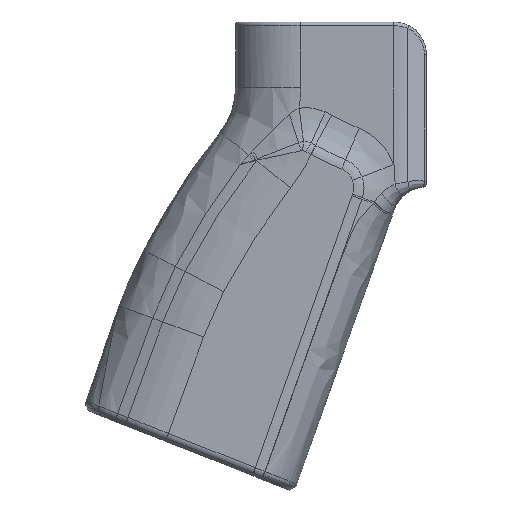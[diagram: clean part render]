
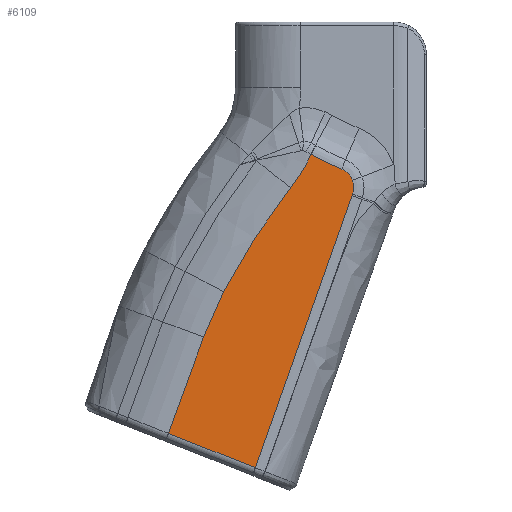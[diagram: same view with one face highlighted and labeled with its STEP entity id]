
A CAD part, left-side view. The second image highlights one B-rep face of the part: STEP entity #6109.
In plain terms, the highlighted planar face has unit normal (-1, 0, 0).
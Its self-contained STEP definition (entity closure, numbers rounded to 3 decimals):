
#480=CIRCLE('',#6562,75.936);
#483=CIRCLE('',#6565,3.889);
#783=FACE_OUTER_BOUND('',#1200,.T.);
#1200=EDGE_LOOP('',(#4482,#4483,#4484,#4485,#4486,#4487,#4488,#4489,#4490,
#4491,#4492,#4493));
#1537=LINE('',#11214,#1730);
#1538=LINE('',#11223,#1731);
#1539=LINE('',#11225,#1732);
#1730=VECTOR('',#7154,10.);
#1731=VECTOR('',#7159,10.);
#1732=VECTOR('',#7160,10.);
#2043=B_SPLINE_CURVE_WITH_KNOTS('',3,(#11066,#11067,#11068,#11069),
 .UNSPECIFIED.,.F.,.F.,(4,4),(-0.965,0.),.UNSPECIFIED.);
#2044=B_SPLINE_CURVE_WITH_KNOTS('',3,(#11088,#11089,#11090,#11091),
 .UNSPECIFIED.,.F.,.F.,(4,4),(-2.413,0.),.UNSPECIFIED.);
#2045=B_SPLINE_CURVE_WITH_KNOTS('',3,(#11109,#11110,#11111,#11112),
 .UNSPECIFIED.,.F.,.F.,(4,4),(-0.596,0.166),
 .UNSPECIFIED.);
#2047=B_SPLINE_CURVE_WITH_KNOTS('',3,(#11156,#11157,#11158,#11159),
 .UNSPECIFIED.,.F.,.F.,(4,4),(0.,0.275),.UNSPECIFIED.);
#2049=B_SPLINE_CURVE_WITH_KNOTS('',3,(#11200,#11201,#11202,#11203),
 .UNSPECIFIED.,.F.,.F.,(4,4),(-0.031,0.),
 .UNSPECIFIED.);
#2052=B_SPLINE_CURVE_WITH_KNOTS('',3,(#11227,#11228,#11229,#11230),
 .UNSPECIFIED.,.F.,.F.,(4,4),(0.,0.002),.UNSPECIFIED.);
#2053=B_SPLINE_CURVE_WITH_KNOTS('',3,(#11231,#11232,#11233,#11234),
 .UNSPECIFIED.,.F.,.F.,(4,4),(0.,0.002),
 .UNSPECIFIED.);
#2586=VERTEX_POINT('',#10744);
#2591=VERTEX_POINT('',#11063);
#2592=VERTEX_POINT('',#11065);
#2593=VERTEX_POINT('',#11087);
#2594=VERTEX_POINT('',#11114);
#2596=VERTEX_POINT('',#11128);
#2599=VERTEX_POINT('',#11150);
#2601=VERTEX_POINT('',#11199);
#2604=VERTEX_POINT('',#11213);
#2606=VERTEX_POINT('',#11222);
#2607=VERTEX_POINT('',#11224);
#2608=VERTEX_POINT('',#11226);
#3273=EDGE_CURVE('',#2591,#2592,#2043,.T.);
#3275=EDGE_CURVE('',#2592,#2593,#2044,.T.);
#3277=EDGE_CURVE('',#2593,#2586,#2045,.T.);
#3278=EDGE_CURVE('',#2586,#2594,#480,.T.);
#3281=EDGE_CURVE('',#2594,#2596,#483,.T.);
#3286=EDGE_CURVE('',#2596,#2599,#2047,.T.);
#3290=EDGE_CURVE('',#2599,#2601,#2049,.T.);
#3294=EDGE_CURVE('',#2601,#2604,#1537,.T.);
#3297=EDGE_CURVE('',#2604,#2606,#1538,.T.);
#3298=EDGE_CURVE('',#2607,#2591,#1539,.T.);
#3299=EDGE_CURVE('',#2608,#2607,#2052,.T.);
#3300=EDGE_CURVE('',#2606,#2608,#2053,.T.);
#4482=ORIENTED_EDGE('',*,*,#3297,.F.);
#4483=ORIENTED_EDGE('',*,*,#3294,.F.);
#4484=ORIENTED_EDGE('',*,*,#3290,.F.);
#4485=ORIENTED_EDGE('',*,*,#3286,.F.);
#4486=ORIENTED_EDGE('',*,*,#3281,.F.);
#4487=ORIENTED_EDGE('',*,*,#3278,.F.);
#4488=ORIENTED_EDGE('',*,*,#3277,.F.);
#4489=ORIENTED_EDGE('',*,*,#3275,.F.);
#4490=ORIENTED_EDGE('',*,*,#3273,.F.);
#4491=ORIENTED_EDGE('',*,*,#3298,.F.);
#4492=ORIENTED_EDGE('',*,*,#3299,.F.);
#4493=ORIENTED_EDGE('',*,*,#3300,.F.);
#5954=PLANE('',#6574);
#6109=ADVANCED_FACE('',(#783),#5954,.T.);
#6562=AXIS2_PLACEMENT_3D('',#11115,#7131,#7132);
#6565=AXIS2_PLACEMENT_3D('',#11129,#7137,#7138);
#6574=AXIS2_PLACEMENT_3D('',#11221,#7157,#7158);
#7131=DIRECTION('center_axis',(-1.,0.,0.));
#7132=DIRECTION('ref_axis',(0.,0.433,-0.901));
#7137=DIRECTION('center_axis',(1.,0.,0.));
#7138=DIRECTION('ref_axis',(0.,-0.72,0.694));
#7154=DIRECTION('',(0.,0.335,-0.942));
#7157=DIRECTION('center_axis',(-1.,0.,0.));
#7158=DIRECTION('ref_axis',(0.,-1.,0.));
#7159=DIRECTION('',(0.,0.93,0.367));
#7160=DIRECTION('',(0.,-0.344,0.939));
#10744=CARTESIAN_POINT('',(-13.29,-131.81,-35.034));
#11063=CARTESIAN_POINT('',(-13.29,-110.892,-70.588));
#11065=CARTESIAN_POINT('',(-13.29,-114.781,-61.762));
#11066=CARTESIAN_POINT('Ctrl Pts',(-13.29,-110.892,
-70.588));
#11067=CARTESIAN_POINT('Ctrl Pts',(-13.29,-111.999,
-67.568));
#11068=CARTESIAN_POINT('Ctrl Pts',(-13.29,-113.299,
-64.618));
#11069=CARTESIAN_POINT('Ctrl Pts',(-13.29,-114.781,
-61.762));
#11087=CARTESIAN_POINT('',(-13.29,-127.852,-41.526));
#11088=CARTESIAN_POINT('Ctrl Pts',(-13.29,-114.781,
-61.762));
#11089=CARTESIAN_POINT('Ctrl Pts',(-13.29,-118.484,
-54.623));
#11090=CARTESIAN_POINT('Ctrl Pts',(-13.29,-122.867,
-47.837));
#11091=CARTESIAN_POINT('Ctrl Pts',(-13.29,-127.852,
-41.526));
#11109=CARTESIAN_POINT('Ctrl Pts',(-13.29,-127.852,
-41.526));
#11110=CARTESIAN_POINT('Ctrl Pts',(-13.29,-129.427,-39.533));
#11111=CARTESIAN_POINT('Ctrl Pts',(-13.29,-130.759,
-37.348));
#11112=CARTESIAN_POINT('Ctrl Pts',(-13.29,-131.81,
-35.034));
#11114=CARTESIAN_POINT('',(-13.29,-137.78,-37.898));
#11115=CARTESIAN_POINT('Origin',(-13.29,-167.611,31.933));
#11128=CARTESIAN_POINT('',(-13.29,-139.883,-40.083));
#11129=CARTESIAN_POINT('Origin',(-13.29,-136.252,-41.474));
#11150=CARTESIAN_POINT('',(-13.29,-139.915,-42.781));
#11156=CARTESIAN_POINT('Ctrl Pts',(-13.29,-139.883,-40.083));
#11157=CARTESIAN_POINT('Ctrl Pts',(-13.29,-140.212,
-40.94));
#11158=CARTESIAN_POINT('Ctrl Pts',(-13.29,-140.222,
-41.916));
#11159=CARTESIAN_POINT('Ctrl Pts',(-13.29,-139.915,
-42.781));
#11199=CARTESIAN_POINT('',(-13.29,-139.811,-43.074));
#11200=CARTESIAN_POINT('Ctrl Pts',(-13.29,-139.915,
-42.781));
#11201=CARTESIAN_POINT('Ctrl Pts',(-13.29,-139.88,
-42.879));
#11202=CARTESIAN_POINT('Ctrl Pts',(-13.29,-139.845,
-42.977));
#11203=CARTESIAN_POINT('Ctrl Pts',(-13.29,-139.811,
-43.074));
#11213=CARTESIAN_POINT('',(-13.29,-120.962,-96.087));
#11214=CARTESIAN_POINT('',(-13.29,-123.761,-88.216));
#11221=CARTESIAN_POINT('Origin',(-13.29,-121.21,-61.501));
#11222=CARTESIAN_POINT('',(-13.29,-104.032,-89.41));
#11223=CARTESIAN_POINT('',(-13.29,-108.831,-91.303));
#11224=CARTESIAN_POINT('',(-13.29,-103.996,-89.395));
#11225=CARTESIAN_POINT('',(-13.29,-110.892,-70.588));
#11226=CARTESIAN_POINT('',(-13.29,-104.011,-89.401));
#11227=CARTESIAN_POINT('Ctrl Pts',(-13.29,-104.011,
-89.401));
#11228=CARTESIAN_POINT('Ctrl Pts',(-13.29,-104.006,
-89.399));
#11229=CARTESIAN_POINT('Ctrl Pts',(-13.29,-104.001,-89.397));
#11230=CARTESIAN_POINT('Ctrl Pts',(-13.29,-103.996,
-89.395));
#11231=CARTESIAN_POINT('Ctrl Pts',(-13.29,-104.032,
-89.41));
#11232=CARTESIAN_POINT('Ctrl Pts',(-13.29,-104.025,-89.407));
#11233=CARTESIAN_POINT('Ctrl Pts',(-13.29,-104.018,
-89.404));
#11234=CARTESIAN_POINT('Ctrl Pts',(-13.29,-104.011,
-89.401));
